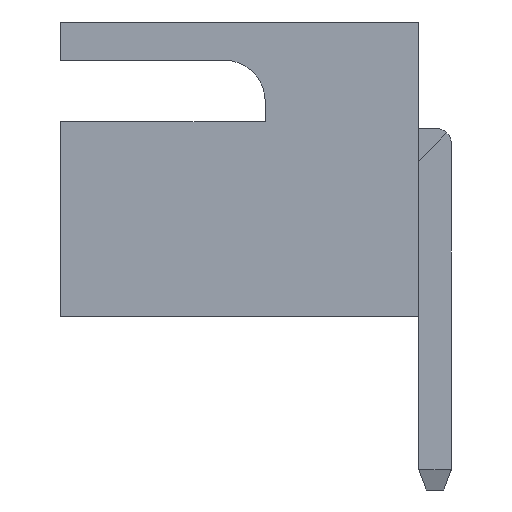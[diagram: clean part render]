
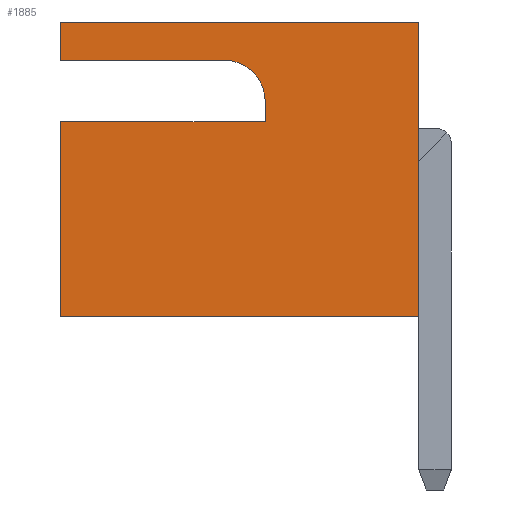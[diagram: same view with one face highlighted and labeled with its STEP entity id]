
A CAD part, left-side view. The second image highlights one B-rep face of the part: STEP entity #1885.
In plain terms, the highlighted planar face has unit normal (-1, 0, 0).
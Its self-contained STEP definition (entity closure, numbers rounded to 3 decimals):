
#43 = VECTOR ( 'NONE', #6351, 1000. ) ;
#199 = CARTESIAN_POINT ( 'NONE',  ( -21.25, 7., 2.125 ) ) ;
#219 = LINE ( 'NONE', #6983, #3490 ) ;
#421 = CARTESIAN_POINT ( 'NONE',  ( -21.25, 7., -2.875 ) ) ;
#731 = ORIENTED_EDGE ( 'NONE', *, *, #1132, .F. ) ;
#758 = CARTESIAN_POINT ( 'NONE',  ( -21.25, 7., 2.875 ) ) ;
#777 = DIRECTION ( 'NONE',  ( 0., 0., -1. ) ) ;
#850 = CARTESIAN_POINT ( 'NONE',  ( -21.25, 7., -2.875 ) ) ;
#870 = CARTESIAN_POINT ( 'NONE',  ( -21.25, 7., -2.875 ) ) ;
#975 = DIRECTION ( 'NONE',  ( 0., 1., 0. ) ) ;
#1132 = EDGE_CURVE ( 'NONE', #1944, #5078, #2604, .T. ) ;
#1408 = CIRCLE ( 'NONE', #2046, 0.8 ) ;
#1425 = DIRECTION ( 'NONE',  ( 0., 0., -1. ) ) ;
#1440 = FACE_OUTER_BOUND ( 'NONE', #4622, .T. ) ;
#1586 = VERTEX_POINT ( 'NONE', #4743 ) ;
#1810 = EDGE_CURVE ( 'NONE', #1944, #5608, #3768, .T. ) ;
#1885 = ADVANCED_FACE ( 'NONE', ( #1440 ), #2079, .F. ) ;
#1944 = VERTEX_POINT ( 'NONE', #199 ) ;
#1990 = EDGE_CURVE ( 'NONE', #5078, #3182, #2158, .T. ) ;
#2046 = AXIS2_PLACEMENT_3D ( 'NONE', #2607, #5094, #1425 ) ;
#2079 = PLANE ( 'NONE',  #3497 ) ;
#2121 = DIRECTION ( 'NONE',  ( 1., 0., 0. ) ) ;
#2125 = ORIENTED_EDGE ( 'NONE', *, *, #4017, .T. ) ;
#2158 = LINE ( 'NONE', #758, #4145 ) ;
#2233 = VECTOR ( 'NONE', #5250, 1000. ) ;
#2422 = DIRECTION ( 'NONE',  ( 0., 0., 1. ) ) ;
#2604 = LINE ( 'NONE', #850, #2233 ) ;
#2607 = CARTESIAN_POINT ( 'NONE',  ( -21.25, 3.8, 1.325 ) ) ;
#2959 = ORIENTED_EDGE ( 'NONE', *, *, #8004, .T. ) ;
#3181 = CARTESIAN_POINT ( 'NONE',  ( -21.25, 0., 2.875 ) ) ;
#3182 = VERTEX_POINT ( 'NONE', #3181 ) ;
#3435 = EDGE_CURVE ( 'NONE', #5608, #7257, #1408, .T. ) ;
#3447 = EDGE_CURVE ( 'NONE', #7257, #7249, #219, .T. ) ;
#3490 = VECTOR ( 'NONE', #777, 1000. ) ;
#3497 = AXIS2_PLACEMENT_3D ( 'NONE', #870, #2121, #7729 ) ;
#3723 = CARTESIAN_POINT ( 'NONE',  ( -21.25, 7., 2.125 ) ) ;
#3768 = LINE ( 'NONE', #3723, #6368 ) ;
#3772 = VECTOR ( 'NONE', #975, 1000. ) ;
#3858 = CARTESIAN_POINT ( 'NONE',  ( -21.25, 0., -2.875 ) ) ;
#4017 = EDGE_CURVE ( 'NONE', #6977, #1586, #7928, .T. ) ;
#4145 = VECTOR ( 'NONE', #7940, 1000. ) ;
#4248 = ORIENTED_EDGE ( 'NONE', *, *, #1990, .F. ) ;
#4319 = ORIENTED_EDGE ( 'NONE', *, *, #3447, .T. ) ;
#4484 = CARTESIAN_POINT ( 'NONE',  ( -21.25, 7., 2.875 ) ) ;
#4539 = CARTESIAN_POINT ( 'NONE',  ( -21.25, 3., 1.325 ) ) ;
#4622 = EDGE_LOOP ( 'NONE', ( #731, #4721, #5903, #4319, #6781, #7303, #2125, #2959, #4248 ) ) ;
#4721 = ORIENTED_EDGE ( 'NONE', *, *, #1810, .T. ) ;
#4743 = CARTESIAN_POINT ( 'NONE',  ( -21.25, 0., -2.875 ) ) ;
#4799 = VERTEX_POINT ( 'NONE', #4973 ) ;
#4973 = CARTESIAN_POINT ( 'NONE',  ( -21.25, 7., 0.925 ) ) ;
#5002 = CARTESIAN_POINT ( 'NONE',  ( -21.25, 3.8, 2.125 ) ) ;
#5078 = VERTEX_POINT ( 'NONE', #4484 ) ;
#5094 = DIRECTION ( 'NONE',  ( 1., 0., 0. ) ) ;
#5250 = DIRECTION ( 'NONE',  ( 0., 0., 1. ) ) ;
#5608 = VERTEX_POINT ( 'NONE', #5002 ) ;
#5620 = EDGE_CURVE ( 'NONE', #6977, #4799, #7462, .T. ) ;
#5903 = ORIENTED_EDGE ( 'NONE', *, *, #3435, .T. ) ;
#6070 = DIRECTION ( 'NONE',  ( 0., -1., 0. ) ) ;
#6207 = DIRECTION ( 'NONE',  ( 0., -1., 0. ) ) ;
#6267 = LINE ( 'NONE', #3858, #43 ) ;
#6351 = DIRECTION ( 'NONE',  ( 0., 0., 1. ) ) ;
#6368 = VECTOR ( 'NONE', #6207, 1000. ) ;
#6526 = LINE ( 'NONE', #6565, #3772 ) ;
#6565 = CARTESIAN_POINT ( 'NONE',  ( -21.25, 7., 0.925 ) ) ;
#6708 = CARTESIAN_POINT ( 'NONE',  ( -21.25, 7., -2.875 ) ) ;
#6781 = ORIENTED_EDGE ( 'NONE', *, *, #7878, .T. ) ;
#6977 = VERTEX_POINT ( 'NONE', #421 ) ;
#6983 = CARTESIAN_POINT ( 'NONE',  ( -21.25, 3., 1.325 ) ) ;
#7021 = VECTOR ( 'NONE', #2422, 1000. ) ;
#7249 = VERTEX_POINT ( 'NONE', #7616 ) ;
#7257 = VERTEX_POINT ( 'NONE', #4539 ) ;
#7303 = ORIENTED_EDGE ( 'NONE', *, *, #5620, .F. ) ;
#7462 = LINE ( 'NONE', #7499, #7021 ) ;
#7499 = CARTESIAN_POINT ( 'NONE',  ( -21.25, 7., -2.875 ) ) ;
#7616 = CARTESIAN_POINT ( 'NONE',  ( -21.25, 3., 0.925 ) ) ;
#7729 = DIRECTION ( 'NONE',  ( 0., 0., -1. ) ) ;
#7789 = VECTOR ( 'NONE', #6070, 1000. ) ;
#7878 = EDGE_CURVE ( 'NONE', #7249, #4799, #6526, .T. ) ;
#7928 = LINE ( 'NONE', #6708, #7789 ) ;
#7940 = DIRECTION ( 'NONE',  ( 0., -1., 0. ) ) ;
#8004 = EDGE_CURVE ( 'NONE', #1586, #3182, #6267, .T. ) ;
